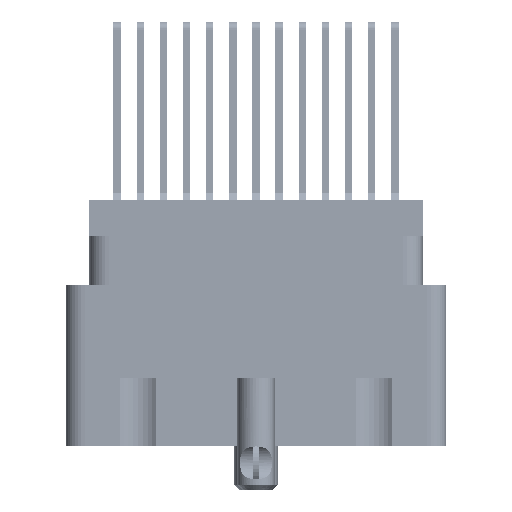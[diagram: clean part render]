
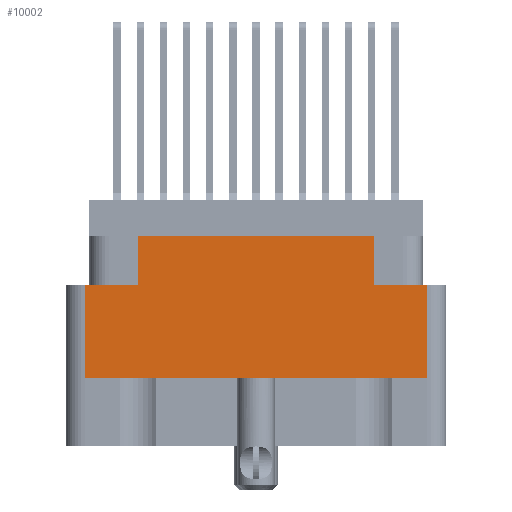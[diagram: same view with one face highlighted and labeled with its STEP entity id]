
A CAD part, left-side view. The second image highlights one B-rep face of the part: STEP entity #10002.
In plain terms, the highlighted planar face has unit normal (-1, 0, 0).
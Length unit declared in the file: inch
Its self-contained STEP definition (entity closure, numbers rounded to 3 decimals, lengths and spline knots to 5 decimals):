
#1035 = CARTESIAN_POINT ( 'NONE',  ( -1.359, -0.555, -0.798 ) ) ;
#1160 = VECTOR ( 'NONE', #74113, 39.37008 ) ;
#3312 = ORIENTED_EDGE ( 'NONE', *, *, #21973, .T. ) ;
#4783 = EDGE_CURVE ( 'NONE', #31005, #79297, #39726, .T. ) ;
#5650 = CARTESIAN_POINT ( 'NONE',  ( -1.359, 0.3825, -0.274 ) ) ;
#6880 = DIRECTION ( 'NONE',  ( 0., 0., 1. ) ) ;
#6928 = PLANE ( 'NONE',  #38782 ) ;
#10002 = ADVANCED_FACE ( 'NONE', ( #44953 ), #6928, .T. ) ;
#10187 = CARTESIAN_POINT ( 'NONE',  ( -1.359, -0.3825, -0.274 ) ) ;
#11496 = EDGE_CURVE ( 'NONE', #68959, #15065, #45872, .T. ) ;
#13106 = CARTESIAN_POINT ( 'NONE',  ( -1.359, -0.555, -0.578 ) ) ;
#13227 = CARTESIAN_POINT ( 'NONE',  ( -1.359, -0.617, -0.798 ) ) ;
#15065 = VERTEX_POINT ( 'NONE', #80425 ) ;
#16109 = ORIENTED_EDGE ( 'NONE', *, *, #11496, .F. ) ;
#17589 = LINE ( 'NONE', #24374, #71799 ) ;
#18011 = DIRECTION ( 'NONE',  ( 0., 0., 1. ) ) ;
#18465 = EDGE_CURVE ( 'NONE', #57623, #18803, #37995, .T. ) ;
#18803 = VERTEX_POINT ( 'NONE', #23868 ) ;
#20524 = LINE ( 'NONE', #5650, #21463 ) ;
#20749 = ORIENTED_EDGE ( 'NONE', *, *, #4783, .T. ) ;
#21463 = VECTOR ( 'NONE', #18011, 39.37008 ) ;
#21973 = EDGE_CURVE ( 'NONE', #51818, #31005, #78986, .T. ) ;
#22678 = CARTESIAN_POINT ( 'NONE',  ( -1.359, 0.555, -0.274 ) ) ;
#23868 = CARTESIAN_POINT ( 'NONE',  ( -1.359, -0.3825, -0.117 ) ) ;
#24137 = DIRECTION ( 'NONE',  ( 0., 0., -1. ) ) ;
#24374 = CARTESIAN_POINT ( 'NONE',  ( -1.359, 0.555, -0.798 ) ) ;
#24993 = DIRECTION ( 'NONE',  ( 0., -1., 0. ) ) ;
#28937 = CARTESIAN_POINT ( 'NONE',  ( -1.359, 0., -0.578 ) ) ;
#31005 = VERTEX_POINT ( 'NONE', #13106 ) ;
#31856 = DIRECTION ( 'NONE',  ( 0., 0., 1. ) ) ;
#32667 = EDGE_CURVE ( 'NONE', #15065, #60652, #20524, .T. ) ;
#36299 = EDGE_CURVE ( 'NONE', #60652, #18803, #78108, .T. ) ;
#37226 = EDGE_CURVE ( 'NONE', #57623, #79297, #68276, .T. ) ;
#37995 = LINE ( 'NONE', #57837, #61720 ) ;
#38782 = AXIS2_PLACEMENT_3D ( 'NONE', #13227, #80182, #75467 ) ;
#39726 = LINE ( 'NONE', #1035, #54603 ) ;
#40508 = DIRECTION ( 'NONE',  ( 0., -1., 0. ) ) ;
#40617 = ORIENTED_EDGE ( 'NONE', *, *, #49407, .T. ) ;
#44953 = FACE_OUTER_BOUND ( 'NONE', #56054, .T. ) ;
#45520 = VECTOR ( 'NONE', #40508, 39.37008 ) ;
#45872 = LINE ( 'NONE', #70237, #77419 ) ;
#49407 = EDGE_CURVE ( 'NONE', #68959, #51818, #17589, .T. ) ;
#50609 = CARTESIAN_POINT ( 'NONE',  ( -1.359, -0.555, -0.274 ) ) ;
#51818 = VERTEX_POINT ( 'NONE', #72479 ) ;
#51919 = ORIENTED_EDGE ( 'NONE', *, *, #36299, .F. ) ;
#52426 = CARTESIAN_POINT ( 'NONE',  ( -1.359, 0., -0.274 ) ) ;
#54603 = VECTOR ( 'NONE', #31856, 39.37008 ) ;
#55348 = ORIENTED_EDGE ( 'NONE', *, *, #18465, .T. ) ;
#56054 = EDGE_LOOP ( 'NONE', ( #16109, #40617, #3312, #20749, #72827, #55348, #51919, #73853 ) ) ;
#57416 = VECTOR ( 'NONE', #24993, 39.37008 ) ;
#57623 = VERTEX_POINT ( 'NONE', #10187 ) ;
#57837 = CARTESIAN_POINT ( 'NONE',  ( -1.359, -0.3825, -0.274 ) ) ;
#60300 = DIRECTION ( 'NONE',  ( 0., -1., 0. ) ) ;
#60652 = VERTEX_POINT ( 'NONE', #72729 ) ;
#61720 = VECTOR ( 'NONE', #6880, 39.37008 ) ;
#66940 = CARTESIAN_POINT ( 'NONE',  ( -1.359, 0.617, -0.117 ) ) ;
#68276 = LINE ( 'NONE', #52426, #45520 ) ;
#68959 = VERTEX_POINT ( 'NONE', #22678 ) ;
#70237 = CARTESIAN_POINT ( 'NONE',  ( -1.359, 0., -0.274 ) ) ;
#71799 = VECTOR ( 'NONE', #24137, 39.37008 ) ;
#72479 = CARTESIAN_POINT ( 'NONE',  ( -1.359, 0.555, -0.578 ) ) ;
#72729 = CARTESIAN_POINT ( 'NONE',  ( -1.359, 0.3825, -0.117 ) ) ;
#72827 = ORIENTED_EDGE ( 'NONE', *, *, #37226, .F. ) ;
#73853 = ORIENTED_EDGE ( 'NONE', *, *, #32667, .F. ) ;
#74113 = DIRECTION ( 'NONE',  ( 0., -1., 0. ) ) ;
#75467 = DIRECTION ( 'NONE',  ( 0., 0., 1. ) ) ;
#77419 = VECTOR ( 'NONE', #60300, 39.37008 ) ;
#78108 = LINE ( 'NONE', #66940, #57416 ) ;
#78986 = LINE ( 'NONE', #28937, #1160 ) ;
#79297 = VERTEX_POINT ( 'NONE', #50609 ) ;
#80182 = DIRECTION ( 'NONE',  ( -1., 0., 0. ) ) ;
#80425 = CARTESIAN_POINT ( 'NONE',  ( -1.359, 0.3825, -0.274 ) ) ;
